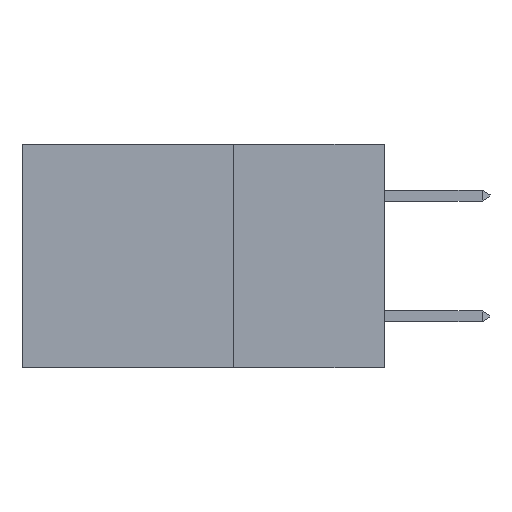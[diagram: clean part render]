
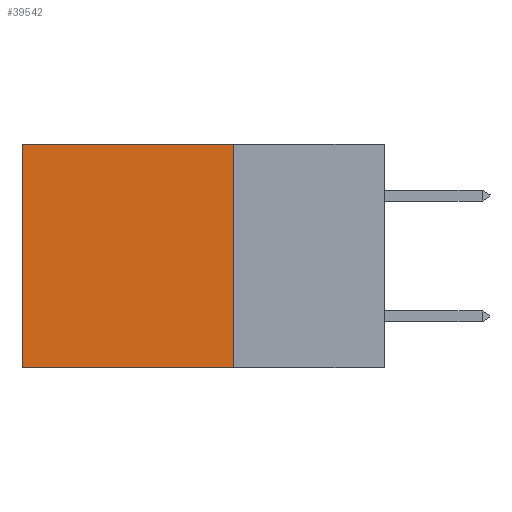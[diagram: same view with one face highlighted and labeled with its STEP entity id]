
A CAD part, left-side view. The second image highlights one B-rep face of the part: STEP entity #39542.
In plain terms, the highlighted planar face has unit normal (-1, 0, 0).
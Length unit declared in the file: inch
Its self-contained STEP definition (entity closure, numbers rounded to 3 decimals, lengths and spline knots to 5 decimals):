
#717 = VECTOR ( 'NONE', #18337, 39.37008 ) ;
#1586 = LINE ( 'NONE', #2463, #19263 ) ;
#2463 = CARTESIAN_POINT ( 'NONE',  ( 0.2875, 0.25, 0. ) ) ;
#2698 = DIRECTION ( 'NONE',  ( 0., 1., 0. ) ) ;
#2765 = VECTOR ( 'NONE', #2698, 39.37008 ) ;
#4398 = ORIENTED_EDGE ( 'NONE', *, *, #16161, .T. ) ;
#4838 = AXIS2_PLACEMENT_3D ( 'NONE', #26573, #19617, #29468 ) ;
#5453 = EDGE_LOOP ( 'NONE', ( #4398, #22816, #11327, #25015 ) ) ;
#6435 = VECTOR ( 'NONE', #23375, 39.37008 ) ;
#7518 = CARTESIAN_POINT ( 'NONE',  ( 0.2875, 0.25, 0. ) ) ;
#11327 = ORIENTED_EDGE ( 'NONE', *, *, #34488, .F. ) ;
#11862 = VERTEX_POINT ( 'NONE', #22917 ) ;
#11919 = VERTEX_POINT ( 'NONE', #7518 ) ;
#15591 = FACE_OUTER_BOUND ( 'NONE', #5453, .T. ) ;
#16161 = EDGE_CURVE ( 'NONE', #11862, #22044, #19909, .T. ) ;
#18337 = DIRECTION ( 'NONE',  ( 0., 0., -1. ) ) ;
#18354 = DIRECTION ( 'NONE',  ( 0., 0., -1. ) ) ;
#19263 = VECTOR ( 'NONE', #18354, 39.37008 ) ;
#19617 = DIRECTION ( 'NONE',  ( 1., 0., 0. ) ) ;
#19909 = LINE ( 'NONE', #31251, #717 ) ;
#22044 = VERTEX_POINT ( 'NONE', #36587 ) ;
#22816 = ORIENTED_EDGE ( 'NONE', *, *, #25464, .F. ) ;
#22917 = CARTESIAN_POINT ( 'NONE',  ( 0.2875, 0.6, 0. ) ) ;
#23254 = PLANE ( 'NONE',  #4838 ) ;
#23375 = DIRECTION ( 'NONE',  ( 0., 1., 0. ) ) ;
#25015 = ORIENTED_EDGE ( 'NONE', *, *, #39827, .T. ) ;
#25464 = EDGE_CURVE ( 'NONE', #30965, #22044, #28633, .T. ) ;
#26573 = CARTESIAN_POINT ( 'NONE',  ( 0.2875, 0.25, 0. ) ) ;
#28633 = LINE ( 'NONE', #32481, #6435 ) ;
#29468 = DIRECTION ( 'NONE',  ( 0., 0., -1. ) ) ;
#30965 = VERTEX_POINT ( 'NONE', #33441 ) ;
#31251 = CARTESIAN_POINT ( 'NONE',  ( 0.2875, 0.6, 0. ) ) ;
#32481 = CARTESIAN_POINT ( 'NONE',  ( 0.2875, 0.25, -0.37 ) ) ;
#33441 = CARTESIAN_POINT ( 'NONE',  ( 0.2875, 0.25, -0.37 ) ) ;
#34488 = EDGE_CURVE ( 'NONE', #11919, #30965, #1586, .T. ) ;
#36587 = CARTESIAN_POINT ( 'NONE',  ( 0.2875, 0.6, -0.37 ) ) ;
#37156 = CARTESIAN_POINT ( 'NONE',  ( 0.2875, 0.25, 0. ) ) ;
#39241 = LINE ( 'NONE', #37156, #2765 ) ;
#39542 = ADVANCED_FACE ( 'NONE', ( #15591 ), #23254, .F. ) ;
#39827 = EDGE_CURVE ( 'NONE', #11919, #11862, #39241, .T. ) ;
